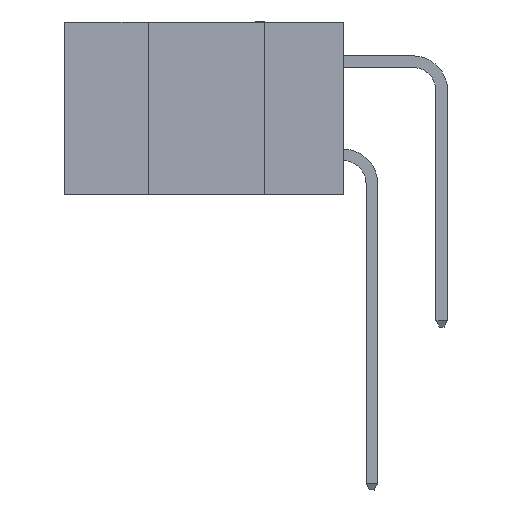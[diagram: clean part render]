
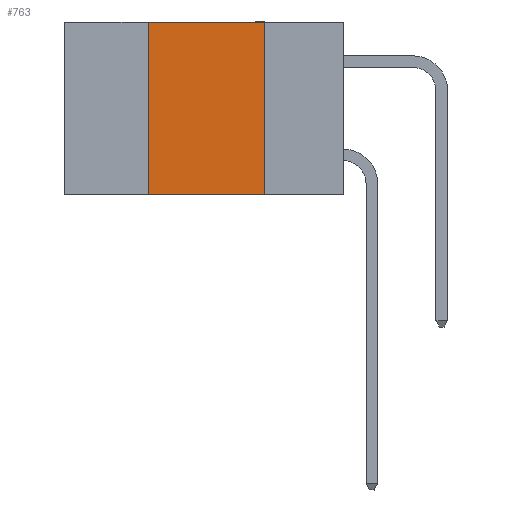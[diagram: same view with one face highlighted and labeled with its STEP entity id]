
A CAD part, left-side view. The second image highlights one B-rep face of the part: STEP entity #763.
In plain terms, the highlighted planar face has unit normal (-1, 0, 0).
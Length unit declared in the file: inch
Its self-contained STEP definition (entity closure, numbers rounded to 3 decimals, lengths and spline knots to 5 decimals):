
#287 = FACE_OUTER_BOUND ( 'NONE', #12832, .T. ) ;
#763 = ADVANCED_FACE ( 'NONE', ( #287 ), #11526, .F. ) ;
#1267 = CARTESIAN_POINT ( 'NONE',  ( 0., 0.42, 0. ) ) ;
#1788 = LINE ( 'NONE', #8720, #13956 ) ;
#2242 = DIRECTION ( 'NONE',  ( 0., 0., -1. ) ) ;
#2935 = VECTOR ( 'NONE', #10808, 39.37008 ) ;
#3777 = DIRECTION ( 'NONE',  ( 0., 0., -1. ) ) ;
#4244 = VERTEX_POINT ( 'NONE', #7162 ) ;
#5241 = CARTESIAN_POINT ( 'NONE',  ( 0., 0.17, -0.37 ) ) ;
#6099 = ORIENTED_EDGE ( 'NONE', *, *, #8994, .F. ) ;
#6499 = CARTESIAN_POINT ( 'NONE',  ( 0., 0.6, 0. ) ) ;
#6984 = VERTEX_POINT ( 'NONE', #5241 ) ;
#7162 = CARTESIAN_POINT ( 'NONE',  ( 0., 0.17, 0. ) ) ;
#8309 = EDGE_CURVE ( 'NONE', #9199, #6984, #1788, .T. ) ;
#8623 = CARTESIAN_POINT ( 'NONE',  ( 0., 0.17, 0. ) ) ;
#8720 = CARTESIAN_POINT ( 'NONE',  ( 0., 0.6, -0.37 ) ) ;
#8994 = EDGE_CURVE ( 'NONE', #4244, #6984, #9994, .T. ) ;
#9199 = VERTEX_POINT ( 'NONE', #19886 ) ;
#9624 = DIRECTION ( 'NONE',  ( 0., -1., 0. ) ) ;
#9994 = LINE ( 'NONE', #8623, #18226 ) ;
#10564 = DIRECTION ( 'NONE',  ( 1., 0., 0. ) ) ;
#10808 = DIRECTION ( 'NONE',  ( 0., 0., 1. ) ) ;
#11526 = PLANE ( 'NONE',  #19573 ) ;
#12815 = VECTOR ( 'NONE', #9624, 39.37008 ) ;
#12832 = EDGE_LOOP ( 'NONE', ( #6099, #16688, #15921, #15698 ) ) ;
#13276 = EDGE_CURVE ( 'NONE', #15855, #4244, #16417, .T. ) ;
#13956 = VECTOR ( 'NONE', #19484, 39.37008 ) ;
#14135 = CARTESIAN_POINT ( 'NONE',  ( 0., 0.6, 0. ) ) ;
#15073 = LINE ( 'NONE', #1267, #2935 ) ;
#15698 = ORIENTED_EDGE ( 'NONE', *, *, #8309, .T. ) ;
#15855 = VERTEX_POINT ( 'NONE', #19079 ) ;
#15921 = ORIENTED_EDGE ( 'NONE', *, *, #19665, .F. ) ;
#16417 = LINE ( 'NONE', #6499, #12815 ) ;
#16688 = ORIENTED_EDGE ( 'NONE', *, *, #13276, .F. ) ;
#18226 = VECTOR ( 'NONE', #3777, 39.37008 ) ;
#19079 = CARTESIAN_POINT ( 'NONE',  ( 0., 0.42, 0. ) ) ;
#19484 = DIRECTION ( 'NONE',  ( 0., -1., 0. ) ) ;
#19573 = AXIS2_PLACEMENT_3D ( 'NONE', #14135, #10564, #2242 ) ;
#19665 = EDGE_CURVE ( 'NONE', #9199, #15855, #15073, .T. ) ;
#19886 = CARTESIAN_POINT ( 'NONE',  ( 0., 0.42, -0.37 ) ) ;
